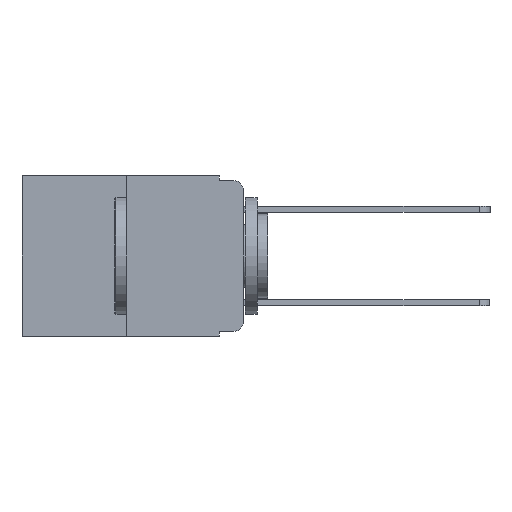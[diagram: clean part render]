
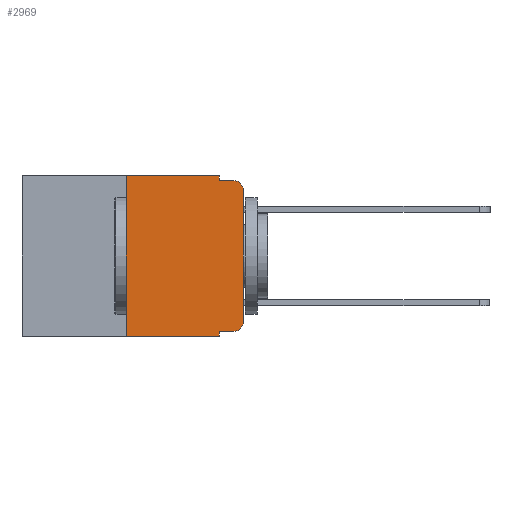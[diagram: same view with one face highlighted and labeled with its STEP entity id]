
A CAD part, left-side view. The second image highlights one B-rep face of the part: STEP entity #2969.
In plain terms, the highlighted planar face has unit normal (-1, 0, 0).
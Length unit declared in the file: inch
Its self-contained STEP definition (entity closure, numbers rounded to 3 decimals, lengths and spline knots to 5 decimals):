
#544 = CARTESIAN_POINT ( 'NONE',  ( 0., 0.02, -0.313 ) ) ;
#552 = VERTEX_POINT ( 'NONE', #5960 ) ;
#576 = CARTESIAN_POINT ( 'NONE',  ( 0., 0.051, 0. ) ) ;
#602 = VERTEX_POINT ( 'NONE', #12664 ) ;
#766 = VERTEX_POINT ( 'NONE', #15009 ) ;
#806 = VERTEX_POINT ( 'NONE', #8368 ) ;
#842 = EDGE_CURVE ( 'NONE', #16330, #13579, #12370, .T. ) ;
#1543 = CIRCLE ( 'NONE', #8413, 0.02 ) ;
#1982 = DIRECTION ( 'NONE',  ( 0., 0., -1. ) ) ;
#2259 = EDGE_CURVE ( 'NONE', #14369, #5249, #5298, .T. ) ;
#2559 = CARTESIAN_POINT ( 'NONE',  ( 0., 0.051, -0.343 ) ) ;
#2573 = CARTESIAN_POINT ( 'NONE',  ( 0., 0.25, 0. ) ) ;
#2969 = ADVANCED_FACE ( 'NONE', ( #11239 ), #15574, .F. ) ;
#2991 = VECTOR ( 'NONE', #17140, 39.37008 ) ;
#3116 = LINE ( 'NONE', #11277, #6682 ) ;
#3144 = ORIENTED_EDGE ( 'NONE', *, *, #842, .F. ) ;
#3249 = DIRECTION ( 'NONE',  ( 0., 0., -1. ) ) ;
#3396 = EDGE_CURVE ( 'NONE', #766, #8772, #3116, .T. ) ;
#3518 = CARTESIAN_POINT ( 'NONE',  ( 0., 0.051, -0.01 ) ) ;
#4059 = EDGE_CURVE ( 'NONE', #806, #5249, #10355, .T. ) ;
#4182 = ORIENTED_EDGE ( 'NONE', *, *, #9718, .T. ) ;
#4371 = VECTOR ( 'NONE', #5609, 39.37008 ) ;
#4596 = CARTESIAN_POINT ( 'NONE',  ( 0., 0.02, -0.03 ) ) ;
#4910 = VECTOR ( 'NONE', #7408, 39.37008 ) ;
#5249 = VERTEX_POINT ( 'NONE', #15475 ) ;
#5298 = LINE ( 'NONE', #5916, #2991 ) ;
#5609 = DIRECTION ( 'NONE',  ( 0., 0., 1. ) ) ;
#5627 = CARTESIAN_POINT ( 'NONE',  ( 0., 0.051, -0.333 ) ) ;
#5796 = CARTESIAN_POINT ( 'NONE',  ( 0., 0.051, 0. ) ) ;
#5916 = CARTESIAN_POINT ( 'NONE',  ( 0., 0.051, -0.01 ) ) ;
#5960 = CARTESIAN_POINT ( 'NONE',  ( 0., 0., -0.313 ) ) ;
#6074 = ORIENTED_EDGE ( 'NONE', *, *, #3396, .T. ) ;
#6342 = VERTEX_POINT ( 'NONE', #9214 ) ;
#6682 = VECTOR ( 'NONE', #6960, 39.37008 ) ;
#6763 = EDGE_CURVE ( 'NONE', #552, #806, #16199, .T. ) ;
#6960 = DIRECTION ( 'NONE',  ( 0., -1., 0. ) ) ;
#7136 = AXIS2_PLACEMENT_3D ( 'NONE', #16054, #15634, #15629 ) ;
#7408 = DIRECTION ( 'NONE',  ( 0., 0., -1. ) ) ;
#7479 = ORIENTED_EDGE ( 'NONE', *, *, #4059, .T. ) ;
#7896 = LINE ( 'NONE', #13488, #4371 ) ;
#8132 = ORIENTED_EDGE ( 'NONE', *, *, #2259, .F. ) ;
#8224 = VECTOR ( 'NONE', #12267, 39.37008 ) ;
#8368 = CARTESIAN_POINT ( 'NONE',  ( 0., 0., -0.03 ) ) ;
#8411 = LINE ( 'NONE', #576, #4910 ) ;
#8413 = AXIS2_PLACEMENT_3D ( 'NONE', #544, #9971, #1982 ) ;
#8772 = VERTEX_POINT ( 'NONE', #2559 ) ;
#8862 = CARTESIAN_POINT ( 'NONE',  ( 0., 0.473, 0. ) ) ;
#9214 = CARTESIAN_POINT ( 'NONE',  ( 0., 0.02, -0.333 ) ) ;
#9235 = VECTOR ( 'NONE', #12209, 39.37008 ) ;
#9718 = EDGE_CURVE ( 'NONE', #6342, #552, #1543, .T. ) ;
#9733 = ORIENTED_EDGE ( 'NONE', *, *, #6763, .T. ) ;
#9971 = DIRECTION ( 'NONE',  ( -1., 0., 0. ) ) ;
#10309 = CARTESIAN_POINT ( 'NONE',  ( 0., 0.051, 0. ) ) ;
#10355 = CIRCLE ( 'NONE', #12351, 0.02 ) ;
#10607 = EDGE_CURVE ( 'NONE', #602, #6342, #15210, .T. ) ;
#10820 = ORIENTED_EDGE ( 'NONE', *, *, #10607, .T. ) ;
#11191 = VECTOR ( 'NONE', #16818, 39.37008 ) ;
#11239 = FACE_OUTER_BOUND ( 'NONE', #15625, .T. ) ;
#11277 = CARTESIAN_POINT ( 'NONE',  ( 0., 0.473, -0.343 ) ) ;
#12209 = DIRECTION ( 'NONE',  ( 0., 0., 1. ) ) ;
#12267 = DIRECTION ( 'NONE',  ( 0., -1., 0. ) ) ;
#12351 = AXIS2_PLACEMENT_3D ( 'NONE', #4596, #12516, #3249 ) ;
#12370 = LINE ( 'NONE', #8862, #15004 ) ;
#12516 = DIRECTION ( 'NONE',  ( -1., 0., 0. ) ) ;
#12664 = CARTESIAN_POINT ( 'NONE',  ( 0., 0.051, -0.333 ) ) ;
#13257 = EDGE_CURVE ( 'NONE', #602, #8772, #15094, .T. ) ;
#13485 = ORIENTED_EDGE ( 'NONE', *, *, #13257, .F. ) ;
#13488 = CARTESIAN_POINT ( 'NONE',  ( 0., 0.25, 0. ) ) ;
#13579 = VERTEX_POINT ( 'NONE', #5796 ) ;
#14090 = ORIENTED_EDGE ( 'NONE', *, *, #14131, .F. ) ;
#14131 = EDGE_CURVE ( 'NONE', #766, #16330, #7896, .T. ) ;
#14369 = VERTEX_POINT ( 'NONE', #3518 ) ;
#15004 = VECTOR ( 'NONE', #16465, 39.37008 ) ;
#15009 = CARTESIAN_POINT ( 'NONE',  ( 0., 0.25, -0.343 ) ) ;
#15094 = LINE ( 'NONE', #10309, #11191 ) ;
#15210 = LINE ( 'NONE', #5627, #8224 ) ;
#15359 = CARTESIAN_POINT ( 'NONE',  ( 0., 0., 0. ) ) ;
#15475 = CARTESIAN_POINT ( 'NONE',  ( 0., 0.02, -0.01 ) ) ;
#15519 = ORIENTED_EDGE ( 'NONE', *, *, #16742, .F. ) ;
#15574 = PLANE ( 'NONE',  #7136 ) ;
#15625 = EDGE_LOOP ( 'NONE', ( #9733, #7479, #8132, #15519, #3144, #14090, #6074, #13485, #10820, #4182 ) ) ;
#15629 = DIRECTION ( 'NONE',  ( 0., 0., -1. ) ) ;
#15634 = DIRECTION ( 'NONE',  ( 1., 0., 0. ) ) ;
#16054 = CARTESIAN_POINT ( 'NONE',  ( 0., 0.473, 0. ) ) ;
#16199 = LINE ( 'NONE', #15359, #9235 ) ;
#16330 = VERTEX_POINT ( 'NONE', #2573 ) ;
#16465 = DIRECTION ( 'NONE',  ( 0., -1., 0. ) ) ;
#16742 = EDGE_CURVE ( 'NONE', #13579, #14369, #8411, .T. ) ;
#16818 = DIRECTION ( 'NONE',  ( 0., 0., -1. ) ) ;
#17140 = DIRECTION ( 'NONE',  ( 0., -1., 0. ) ) ;
